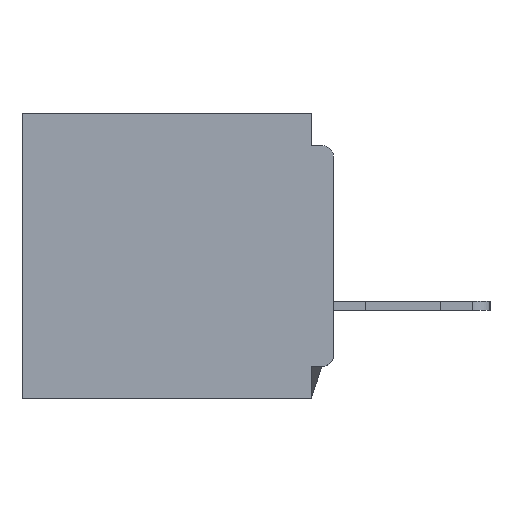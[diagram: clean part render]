
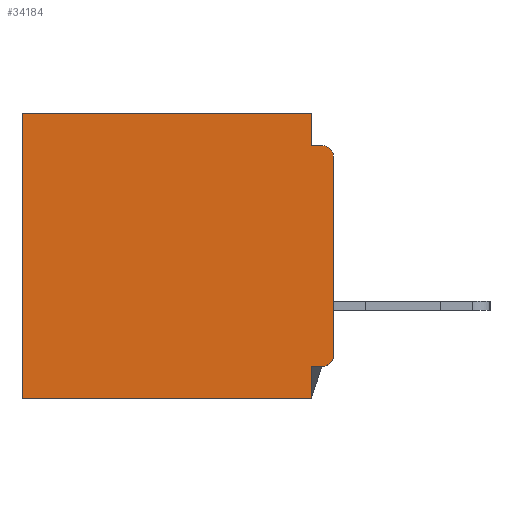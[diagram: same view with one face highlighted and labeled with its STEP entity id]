
A CAD part, left-side view. The second image highlights one B-rep face of the part: STEP entity #34184.
In plain terms, the highlighted planar face has unit normal (-1, 0, 0).
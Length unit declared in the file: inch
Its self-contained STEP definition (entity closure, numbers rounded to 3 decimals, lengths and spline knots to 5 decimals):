
#1939 = PLANE ( 'NONE',  #44785 ) ;
#2051 = VERTEX_POINT ( 'NONE', #4070 ) ;
#2085 = LINE ( 'NONE', #13701, #30627 ) ;
#2426 = ORIENTED_EDGE ( 'NONE', *, *, #24732, .F. ) ;
#3075 = CARTESIAN_POINT ( 'NONE',  ( 0.3, 0.015, -0.06 ) ) ;
#3599 = VERTEX_POINT ( 'NONE', #7408 ) ;
#3637 = VECTOR ( 'NONE', #42651, 39.37008 ) ;
#3750 = EDGE_CURVE ( 'NONE', #3599, #25401, #36478, .T. ) ;
#4070 = CARTESIAN_POINT ( 'NONE',  ( 0.3, 0.437, 0. ) ) ;
#5959 = LINE ( 'NONE', #43666, #24616 ) ;
#6240 = VECTOR ( 'NONE', #39533, 39.37008 ) ;
#6834 = DIRECTION ( 'NONE',  ( 0., 0., -1. ) ) ;
#7163 = ORIENTED_EDGE ( 'NONE', *, *, #22022, .T. ) ;
#7174 = CARTESIAN_POINT ( 'NONE',  ( 0.3, 0.015, -0.34 ) ) ;
#7408 = CARTESIAN_POINT ( 'NONE',  ( 0.3, 0.031, -0.4 ) ) ;
#7542 = VERTEX_POINT ( 'NONE', #10865 ) ;
#7958 = VERTEX_POINT ( 'NONE', #31950 ) ;
#9440 = EDGE_LOOP ( 'NONE', ( #12953, #47107, #28636, #2426, #35633, #7163, #40248, #26987, #18293, #22598 ) ) ;
#9638 = DIRECTION ( 'NONE',  ( 0., 0., -1. ) ) ;
#10167 = AXIS2_PLACEMENT_3D ( 'NONE', #7174, #33188, #10944 ) ;
#10865 = CARTESIAN_POINT ( 'NONE',  ( 0.3, 0.031, 0. ) ) ;
#10944 = DIRECTION ( 'NONE',  ( 0., 0., -1. ) ) ;
#11597 = LINE ( 'NONE', #16007, #32513 ) ;
#11748 = AXIS2_PLACEMENT_3D ( 'NONE', #3075, #29119, #6834 ) ;
#12953 = ORIENTED_EDGE ( 'NONE', *, *, #32909, .F. ) ;
#13020 = EDGE_CURVE ( 'NONE', #18505, #20674, #2085, .T. ) ;
#13701 = CARTESIAN_POINT ( 'NONE',  ( 0.3, 0., -0.045 ) ) ;
#13769 = CARTESIAN_POINT ( 'NONE',  ( 0.3, 0., -0.06 ) ) ;
#13815 = DIRECTION ( 'NONE',  ( 0., 1., 0. ) ) ;
#14210 = VERTEX_POINT ( 'NONE', #13769 ) ;
#14857 = DIRECTION ( 'NONE',  ( 0., 0., -1. ) ) ;
#16007 = CARTESIAN_POINT ( 'NONE',  ( 0.3, 0., 0. ) ) ;
#16290 = CARTESIAN_POINT ( 'NONE',  ( 0.3, 0.031, -0.355 ) ) ;
#18293 = ORIENTED_EDGE ( 'NONE', *, *, #41206, .F. ) ;
#18505 = VERTEX_POINT ( 'NONE', #36167 ) ;
#20674 = VERTEX_POINT ( 'NONE', #29963 ) ;
#21490 = DIRECTION ( 'NONE',  ( 0., 0., -1. ) ) ;
#21669 = CARTESIAN_POINT ( 'NONE',  ( 0.3, 0.437, -0.4 ) ) ;
#22022 = EDGE_CURVE ( 'NONE', #2051, #25401, #5959, .T. ) ;
#22598 = ORIENTED_EDGE ( 'NONE', *, *, #23877, .T. ) ;
#23877 = EDGE_CURVE ( 'NONE', #46251, #7958, #24989, .T. ) ;
#24616 = VECTOR ( 'NONE', #21490, 39.37008 ) ;
#24732 = EDGE_CURVE ( 'NONE', #7542, #18505, #27201, .T. ) ;
#24989 = CIRCLE ( 'NONE', #10167, 0.015 ) ;
#25401 = VERTEX_POINT ( 'NONE', #21669 ) ;
#25899 = CARTESIAN_POINT ( 'NONE',  ( 0.3, 0.031, -0.4 ) ) ;
#26286 = CARTESIAN_POINT ( 'NONE',  ( 0.3, 0., -0.355 ) ) ;
#26736 = CARTESIAN_POINT ( 'NONE',  ( 0.3, 0., -0.4 ) ) ;
#26782 = VECTOR ( 'NONE', #44847, 39.37008 ) ;
#26964 = VECTOR ( 'NONE', #14857, 39.37008 ) ;
#26987 = ORIENTED_EDGE ( 'NONE', *, *, #30581, .F. ) ;
#27201 = LINE ( 'NONE', #35865, #6240 ) ;
#28165 = CARTESIAN_POINT ( 'NONE',  ( 0.3, 0., -0.4 ) ) ;
#28636 = ORIENTED_EDGE ( 'NONE', *, *, #13020, .F. ) ;
#28871 = EDGE_CURVE ( 'NONE', #14210, #20674, #47952, .T. ) ;
#29119 = DIRECTION ( 'NONE',  ( -1., 0., 0. ) ) ;
#29123 = LINE ( 'NONE', #26286, #26782 ) ;
#29713 = FACE_OUTER_BOUND ( 'NONE', #9440, .T. ) ;
#29963 = CARTESIAN_POINT ( 'NONE',  ( 0.3, 0.015, -0.045 ) ) ;
#30581 = EDGE_CURVE ( 'NONE', #46719, #3599, #36869, .T. ) ;
#30627 = VECTOR ( 'NONE', #32208, 39.37008 ) ;
#31552 = CARTESIAN_POINT ( 'NONE',  ( 0.3, 0., -0.4 ) ) ;
#31908 = DIRECTION ( 'NONE',  ( 1., 0., 0. ) ) ;
#31950 = CARTESIAN_POINT ( 'NONE',  ( 0.3, 0., -0.34 ) ) ;
#32208 = DIRECTION ( 'NONE',  ( 0., -1., 0. ) ) ;
#32513 = VECTOR ( 'NONE', #38205, 39.37008 ) ;
#32909 = EDGE_CURVE ( 'NONE', #14210, #7958, #43139, .T. ) ;
#33188 = DIRECTION ( 'NONE',  ( -1., 0., 0. ) ) ;
#34184 = ADVANCED_FACE ( 'NONE', ( #29713 ), #1939, .F. ) ;
#35239 = EDGE_CURVE ( 'NONE', #7542, #2051, #11597, .T. ) ;
#35633 = ORIENTED_EDGE ( 'NONE', *, *, #35239, .T. ) ;
#35865 = CARTESIAN_POINT ( 'NONE',  ( 0.3, 0.031, 0. ) ) ;
#36167 = CARTESIAN_POINT ( 'NONE',  ( 0.3, 0.031, -0.045 ) ) ;
#36478 = LINE ( 'NONE', #26736, #43932 ) ;
#36869 = LINE ( 'NONE', #25899, #26964 ) ;
#38205 = DIRECTION ( 'NONE',  ( 0., 1., 0. ) ) ;
#39533 = DIRECTION ( 'NONE',  ( 0., 0., -1. ) ) ;
#40248 = ORIENTED_EDGE ( 'NONE', *, *, #3750, .F. ) ;
#41206 = EDGE_CURVE ( 'NONE', #46251, #46719, #29123, .T. ) ;
#42651 = DIRECTION ( 'NONE',  ( 0., 0., -1. ) ) ;
#43139 = LINE ( 'NONE', #31552, #3637 ) ;
#43666 = CARTESIAN_POINT ( 'NONE',  ( 0.3, 0.437, -0.4 ) ) ;
#43890 = CARTESIAN_POINT ( 'NONE',  ( 0.3, 0.015, -0.355 ) ) ;
#43932 = VECTOR ( 'NONE', #13815, 39.37008 ) ;
#44785 = AXIS2_PLACEMENT_3D ( 'NONE', #28165, #31908, #9638 ) ;
#44847 = DIRECTION ( 'NONE',  ( 0., 1., 0. ) ) ;
#46251 = VERTEX_POINT ( 'NONE', #43890 ) ;
#46719 = VERTEX_POINT ( 'NONE', #16290 ) ;
#47107 = ORIENTED_EDGE ( 'NONE', *, *, #28871, .T. ) ;
#47952 = CIRCLE ( 'NONE', #11748, 0.015 ) ;
